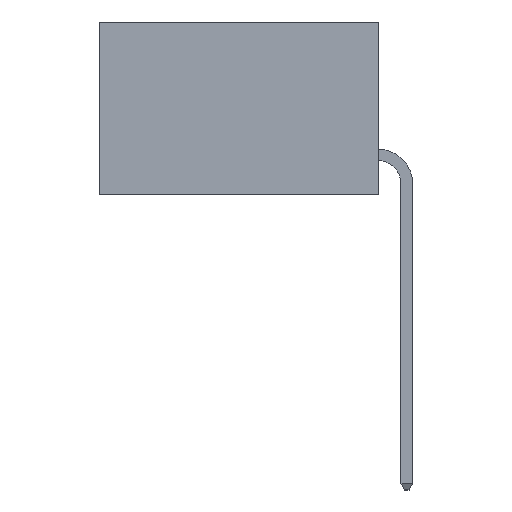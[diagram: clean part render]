
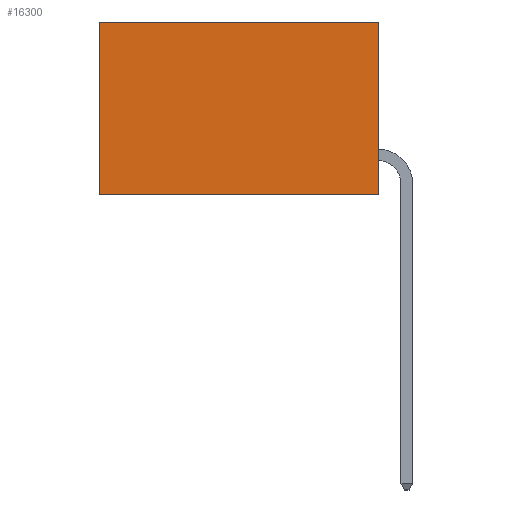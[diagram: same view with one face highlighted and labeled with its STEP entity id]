
A CAD part, left-side view. The second image highlights one B-rep face of the part: STEP entity #16300.
In plain terms, the highlighted planar face has unit normal (-1, 0, 0).
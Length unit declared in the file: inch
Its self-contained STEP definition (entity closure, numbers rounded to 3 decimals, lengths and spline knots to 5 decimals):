
#782 = EDGE_LOOP ( 'NONE', ( #14557, #15139, #6749, #1274 ) ) ;
#1262 = VECTOR ( 'NONE', #10251, 39.37008 ) ;
#1274 = ORIENTED_EDGE ( 'NONE', *, *, #19824, .T. ) ;
#1987 = EDGE_CURVE ( 'NONE', #16385, #19385, #11725, .T. ) ;
#2496 = DIRECTION ( 'NONE',  ( 1., 0., 0. ) ) ;
#3149 = EDGE_CURVE ( 'NONE', #8109, #4652, #15558, .T. ) ;
#3365 = DIRECTION ( 'NONE',  ( 0., 1., 0. ) ) ;
#4652 = VERTEX_POINT ( 'NONE', #24987 ) ;
#4805 = AXIS2_PLACEMENT_3D ( 'NONE', #24414, #2496, #16635 ) ;
#6335 = VECTOR ( 'NONE', #20587, 39.37008 ) ;
#6749 = ORIENTED_EDGE ( 'NONE', *, *, #3149, .F. ) ;
#8109 = VERTEX_POINT ( 'NONE', #19086 ) ;
#9467 = DIRECTION ( 'NONE',  ( 0., 0., -1. ) ) ;
#10219 = VECTOR ( 'NONE', #9467, 39.37008 ) ;
#10251 = DIRECTION ( 'NONE',  ( 0., 1., 0. ) ) ;
#10496 = CARTESIAN_POINT ( 'NONE',  ( 0.2615, 0., -0.37 ) ) ;
#10498 = EDGE_CURVE ( 'NONE', #4652, #19385, #18329, .T. ) ;
#11670 = FACE_OUTER_BOUND ( 'NONE', #782, .T. ) ;
#11725 = LINE ( 'NONE', #15941, #6335 ) ;
#12441 = VECTOR ( 'NONE', #3365, 39.37008 ) ;
#13362 = CARTESIAN_POINT ( 'NONE',  ( 0.2615, 0., -0.37 ) ) ;
#14557 = ORIENTED_EDGE ( 'NONE', *, *, #1987, .T. ) ;
#14639 = PLANE ( 'NONE',  #4805 ) ;
#15139 = ORIENTED_EDGE ( 'NONE', *, *, #10498, .F. ) ;
#15558 = LINE ( 'NONE', #10496, #10219 ) ;
#15941 = CARTESIAN_POINT ( 'NONE',  ( 0.2615, 0.6, -0.37 ) ) ;
#16300 = ADVANCED_FACE ( 'NONE', ( #11670 ), #14639, .F. ) ;
#16385 = VERTEX_POINT ( 'NONE', #18785 ) ;
#16635 = DIRECTION ( 'NONE',  ( 0., 0., -1. ) ) ;
#16796 = LINE ( 'NONE', #22129, #1262 ) ;
#16930 = CARTESIAN_POINT ( 'NONE',  ( 0.2615, 0.6, -0.37 ) ) ;
#18329 = LINE ( 'NONE', #13362, #12441 ) ;
#18785 = CARTESIAN_POINT ( 'NONE',  ( 0.2615, 0.6, 0. ) ) ;
#19086 = CARTESIAN_POINT ( 'NONE',  ( 0.2615, 0., 0. ) ) ;
#19385 = VERTEX_POINT ( 'NONE', #16930 ) ;
#19824 = EDGE_CURVE ( 'NONE', #8109, #16385, #16796, .T. ) ;
#20587 = DIRECTION ( 'NONE',  ( 0., 0., -1. ) ) ;
#22129 = CARTESIAN_POINT ( 'NONE',  ( 0.2615, 0., 0. ) ) ;
#24414 = CARTESIAN_POINT ( 'NONE',  ( 0.2615, 0., -0.37 ) ) ;
#24987 = CARTESIAN_POINT ( 'NONE',  ( 0.2615, 0., -0.37 ) ) ;
